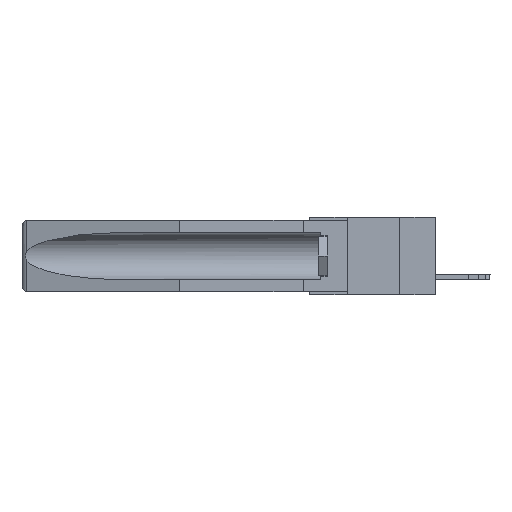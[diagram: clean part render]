
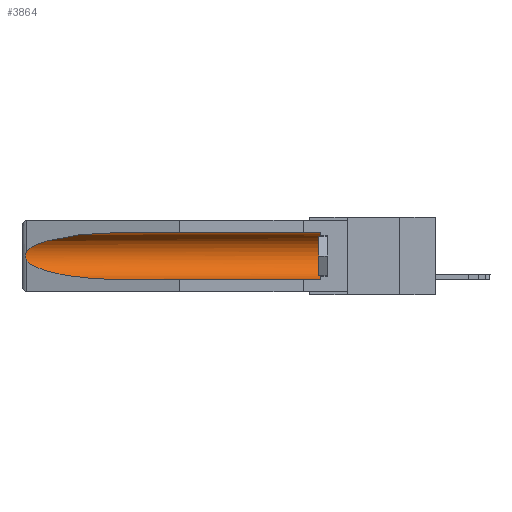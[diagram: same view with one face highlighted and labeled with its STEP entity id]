
A CAD part, left-side view. The second image highlights one B-rep face of the part: STEP entity #3864.
In plain terms, the highlighted cylindrical face has radius 2.857 mm (diameter 5.715 mm), a partial arc.
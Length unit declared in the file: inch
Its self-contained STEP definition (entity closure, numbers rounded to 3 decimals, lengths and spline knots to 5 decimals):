
#83 =( BOUNDED_CURVE ( )  B_SPLINE_CURVE ( 3, ( #5032, #4756, #7138, #22089 ),
 .UNSPECIFIED., .F., .F. ) 
 B_SPLINE_CURVE_WITH_KNOTS ( ( 4, 4 ),
 ( 0.1948, 1.5708 ),
 .UNSPECIFIED. ) 
 CURVE ( )  GEOMETRIC_REPRESENTATION_ITEM ( )  RATIONAL_B_SPLINE_CURVE ( ( 1., 0.848, 0.848, 1. ) ) 
 REPRESENTATION_ITEM ( '' )  );
#661 = CARTESIAN_POINT ( 'NONE',  ( 0.26537, 1.52718, -0.14972 ) ) ;
#1235 = FACE_OUTER_BOUND ( 'NONE', #13315, .T. ) ;
#1312 = DIRECTION ( 'NONE',  ( 0., 1., 0. ) ) ;
#1382 = DIRECTION ( 'NONE',  ( 0., 1., 0. ) ) ;
#1455 = AXIS2_PLACEMENT_3D ( 'NONE', #22705, #1382, #18067 ) ;
#2301 = CARTESIAN_POINT ( 'NONE',  ( 0.155, 1.07973, -0.284 ) ) ;
#2744 = VECTOR ( 'NONE', #11422, 39.37008 ) ;
#3026 = CARTESIAN_POINT ( 'NONE',  ( 0.26597, 1.5296, -0.19026 ) ) ;
#3106 = EDGE_CURVE ( 'NONE', #9893, #17072, #25910, .T. ) ;
#3405 = CARTESIAN_POINT ( 'NONE',  ( 0.155, 0.126, -0.284 ) ) ;
#3864 = ADVANCED_FACE ( 'NONE', ( #1235 ), #9941, .F. ) ;
#4533 = ORIENTED_EDGE ( 'NONE', *, *, #12287, .T. ) ;
#4756 = CARTESIAN_POINT ( 'NONE',  ( 0.25451, 1.48313, -0.24835 ) ) ;
#5032 = CARTESIAN_POINT ( 'NONE',  ( 0.26537, 1.52718, -0.19328 ) ) ;
#6321 = EDGE_CURVE ( 'NONE', #8166, #16554, #9768, .T. ) ;
#6916 = CARTESIAN_POINT ( 'NONE',  ( 0.155, 1.07973, -0.059 ) ) ;
#7138 = CARTESIAN_POINT ( 'NONE',  ( 0.21114, 1.30732, -0.284 ) ) ;
#8166 = VERTEX_POINT ( 'NONE', #15617 ) ;
#8365 = AXIS2_PLACEMENT_3D ( 'NONE', #22699, #17453, #13857 ) ;
#9129 = CARTESIAN_POINT ( 'NONE',  ( 0.25451, 1.48313, -0.09465 ) ) ;
#9228 = CARTESIAN_POINT ( 'NONE',  ( 0.155, 1.07973, -0.059 ) ) ;
#9251 = EDGE_CURVE ( 'NONE', #16448, #17072, #83, .T. ) ;
#9604 = CARTESIAN_POINT ( 'NONE',  ( 0.155, -0.30754, -0.284 ) ) ;
#9768 = LINE ( 'NONE', #13666, #2744 ) ;
#9893 = VERTEX_POINT ( 'NONE', #3405 ) ;
#9941 = CYLINDRICAL_SURFACE ( 'NONE', #1455, 0.1125 ) ;
#9992 =( BOUNDED_CURVE ( )  B_SPLINE_CURVE ( 3, ( #9228, #10827, #9129, #11638 ),
 .UNSPECIFIED., .F., .T. ) 
 B_SPLINE_CURVE_WITH_KNOTS ( ( 4, 4 ),
 ( 4.71239, 6.08839 ),
 .UNSPECIFIED. ) 
 CURVE ( )  GEOMETRIC_REPRESENTATION_ITEM ( )  RATIONAL_B_SPLINE_CURVE ( ( 1., 0.848, 0.848, 1. ) ) 
 REPRESENTATION_ITEM ( '' )  );
#10827 = CARTESIAN_POINT ( 'NONE',  ( 0.21114, 1.30732, -0.059 ) ) ;
#11422 = DIRECTION ( 'NONE',  ( 0., 1., 0. ) ) ;
#11638 = CARTESIAN_POINT ( 'NONE',  ( 0.26537, 1.52718, -0.14972 ) ) ;
#11796 = CARTESIAN_POINT ( 'NONE',  ( 0.26537, 1.52718, -0.19328 ) ) ;
#12287 = EDGE_CURVE ( 'NONE', #9893, #8166, #19429, .T. ) ;
#13315 = EDGE_LOOP ( 'NONE', ( #16085, #24618, #14697, #17217, #4533, #22841 ) ) ;
#13666 = CARTESIAN_POINT ( 'NONE',  ( 0.155, -0.30754, -0.059 ) ) ;
#13857 = DIRECTION ( 'NONE',  ( 0., 0., 1. ) ) ;
#14697 = ORIENTED_EDGE ( 'NONE', *, *, #9251, .T. ) ;
#15297 = B_SPLINE_CURVE_WITH_KNOTS ( 'NONE', 3,
 ( #20185, #26699, #15902, #20280, #20096, #24544, #22142, #24182, #3026, #11796 ),
 .UNSPECIFIED., .F., .F.,
 ( 4, 2, 2, 2, 4 ),
 ( 0., 0.00029, 0.00058, 0.00087, 0.00117 ),
 .UNSPECIFIED. ) ;
#15617 = CARTESIAN_POINT ( 'NONE',  ( 0.155, 0.126, -0.059 ) ) ;
#15902 = CARTESIAN_POINT ( 'NONE',  ( 0.26654, 1.53092, -0.15636 ) ) ;
#16085 = ORIENTED_EDGE ( 'NONE', *, *, #20821, .T. ) ;
#16193 = CARTESIAN_POINT ( 'NONE',  ( 0.26537, 1.52718, -0.19328 ) ) ;
#16353 = VERTEX_POINT ( 'NONE', #661 ) ;
#16448 = VERTEX_POINT ( 'NONE', #16193 ) ;
#16554 = VERTEX_POINT ( 'NONE', #6916 ) ;
#17072 = VERTEX_POINT ( 'NONE', #2301 ) ;
#17217 = ORIENTED_EDGE ( 'NONE', *, *, #3106, .F. ) ;
#17453 = DIRECTION ( 'NONE',  ( 0., -1., 0. ) ) ;
#18067 = DIRECTION ( 'NONE',  ( 0., 0., 1. ) ) ;
#19429 = CIRCLE ( 'NONE', #8365, 0.1125 ) ;
#19598 = VECTOR ( 'NONE', #1312, 39.37008 ) ;
#20096 = CARTESIAN_POINT ( 'NONE',  ( 0.2675, 1.53308, -0.16763 ) ) ;
#20185 = CARTESIAN_POINT ( 'NONE',  ( 0.26537, 1.52718, -0.14972 ) ) ;
#20280 = CARTESIAN_POINT ( 'NONE',  ( 0.2673, 1.5327, -0.16383 ) ) ;
#20821 = EDGE_CURVE ( 'NONE', #16554, #16353, #9992, .T. ) ;
#22089 = CARTESIAN_POINT ( 'NONE',  ( 0.155, 1.07973, -0.284 ) ) ;
#22142 = CARTESIAN_POINT ( 'NONE',  ( 0.2673, 1.53269, -0.17917 ) ) ;
#22699 = CARTESIAN_POINT ( 'NONE',  ( 0.155, 0.126, -0.1715 ) ) ;
#22705 = CARTESIAN_POINT ( 'NONE',  ( 0.155, -0.30754, -0.1715 ) ) ;
#22841 = ORIENTED_EDGE ( 'NONE', *, *, #6321, .T. ) ;
#24182 = CARTESIAN_POINT ( 'NONE',  ( 0.26655, 1.53094, -0.18657 ) ) ;
#24544 = CARTESIAN_POINT ( 'NONE',  ( 0.2675, 1.53308, -0.17534 ) ) ;
#24618 = ORIENTED_EDGE ( 'NONE', *, *, #25552, .T. ) ;
#25552 = EDGE_CURVE ( 'NONE', #16353, #16448, #15297, .T. ) ;
#25910 = LINE ( 'NONE', #9604, #19598 ) ;
#26699 = CARTESIAN_POINT ( 'NONE',  ( 0.26597, 1.52961, -0.15275 ) ) ;
